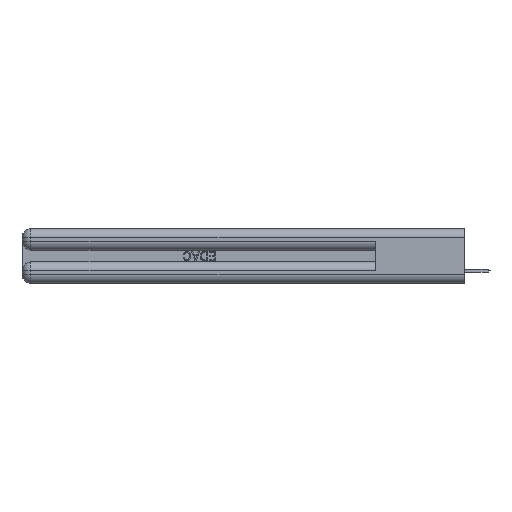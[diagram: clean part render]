
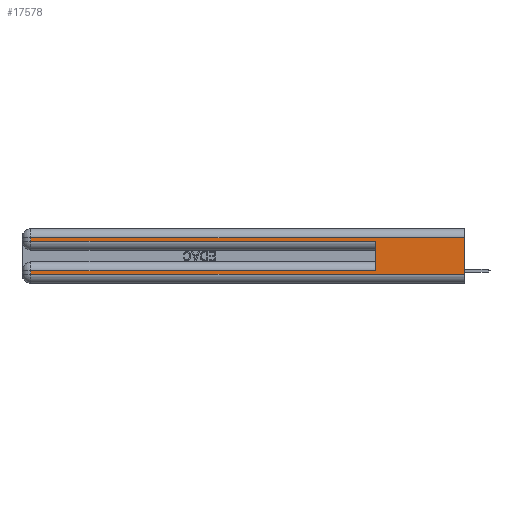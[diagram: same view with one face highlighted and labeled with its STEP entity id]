
A CAD part, left-side view. The second image highlights one B-rep face of the part: STEP entity #17578.
In plain terms, the highlighted planar face has unit normal (-1, 0, 0).
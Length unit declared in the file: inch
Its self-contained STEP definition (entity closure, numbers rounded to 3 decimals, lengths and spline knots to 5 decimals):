
#27 = VERTEX_POINT ( 'NONE', #25261 ) ;
#1653 = EDGE_CURVE ( 'NONE', #27, #19841, #10966, .T. ) ;
#1746 = EDGE_CURVE ( 'NONE', #1785, #27, #41986, .T. ) ;
#1785 = VERTEX_POINT ( 'NONE', #32756 ) ;
#2063 = VECTOR ( 'NONE', #39523, 39.37008 ) ;
#3125 = CARTESIAN_POINT ( 'NONE',  ( 0., 0., 0.06 ) ) ;
#3325 = DIRECTION ( 'NONE',  ( 0., 1., 0. ) ) ;
#3582 = CARTESIAN_POINT ( 'NONE',  ( 0., 0., 0.06 ) ) ;
#3936 = CARTESIAN_POINT ( 'NONE',  ( 0., 0., 0.31 ) ) ;
#4228 = EDGE_CURVE ( 'NONE', #26138, #29445, #43855, .T. ) ;
#4546 = FACE_OUTER_BOUND ( 'NONE', #14068, .T. ) ;
#5869 = CARTESIAN_POINT ( 'NONE',  ( 0., 0., 0.37 ) ) ;
#6634 = DIRECTION ( 'NONE',  ( 0., -1., 0. ) ) ;
#8595 = LINE ( 'NONE', #5869, #16922 ) ;
#8625 = CARTESIAN_POINT ( 'NONE',  ( 0., 0.6, 0.085 ) ) ;
#8633 = CARTESIAN_POINT ( 'NONE',  ( 0., 0., 0.285 ) ) ;
#8970 = VECTOR ( 'NONE', #6634, 39.37008 ) ;
#10349 = CARTESIAN_POINT ( 'NONE',  ( 0., 0.6, 0.145 ) ) ;
#10935 = ORIENTED_EDGE ( 'NONE', *, *, #47325, .T. ) ;
#10966 = LINE ( 'NONE', #22356, #48543 ) ;
#11278 = DIRECTION ( 'NONE',  ( 0., 0., -1. ) ) ;
#11519 = VECTOR ( 'NONE', #3325, 39.37008 ) ;
#12104 = LINE ( 'NONE', #36018, #2063 ) ;
#12710 = LINE ( 'NONE', #32894, #11519 ) ;
#13672 = VERTEX_POINT ( 'NONE', #29238 ) ;
#13933 = ORIENTED_EDGE ( 'NONE', *, *, #4228, .F. ) ;
#14068 = EDGE_LOOP ( 'NONE', ( #26017, #23106, #38516, #34493, #13933, #10935, #15301, #30255 ) ) ;
#14359 = LINE ( 'NONE', #3582, #8970 ) ;
#15072 = AXIS2_PLACEMENT_3D ( 'NONE', #21976, #41935, #11278 ) ;
#15301 = ORIENTED_EDGE ( 'NONE', *, *, #18560, .T. ) ;
#16390 = VECTOR ( 'NONE', #22319, 39.37008 ) ;
#16622 = EDGE_CURVE ( 'NONE', #19841, #29445, #30000, .T. ) ;
#16922 = VECTOR ( 'NONE', #24989, 39.37008 ) ;
#17297 = DIRECTION ( 'NONE',  ( 0., -1., 0. ) ) ;
#17509 = CARTESIAN_POINT ( 'NONE',  ( 0., 0.6, 0.285 ) ) ;
#17578 = ADVANCED_FACE ( 'NONE', ( #4546 ), #44819, .F. ) ;
#18560 = EDGE_CURVE ( 'NONE', #13672, #44566, #12104, .T. ) ;
#19841 = VERTEX_POINT ( 'NONE', #37607 ) ;
#19845 = VECTOR ( 'NONE', #17297, 39.37008 ) ;
#21607 = CARTESIAN_POINT ( 'NONE',  ( 0., 2.94, 0.06 ) ) ;
#21976 = CARTESIAN_POINT ( 'NONE',  ( 0., 0., 0.37 ) ) ;
#22319 = DIRECTION ( 'NONE',  ( 0., 0., 1. ) ) ;
#22356 = CARTESIAN_POINT ( 'NONE',  ( 0., 2.94, 0.37 ) ) ;
#23106 = ORIENTED_EDGE ( 'NONE', *, *, #1746, .T. ) ;
#23675 = VERTEX_POINT ( 'NONE', #3125 ) ;
#24989 = DIRECTION ( 'NONE',  ( 0., 0., -1. ) ) ;
#25261 = CARTESIAN_POINT ( 'NONE',  ( 0., 2.94, 0.31 ) ) ;
#26017 = ORIENTED_EDGE ( 'NONE', *, *, #29095, .F. ) ;
#26138 = VERTEX_POINT ( 'NONE', #8625 ) ;
#29095 = EDGE_CURVE ( 'NONE', #1785, #23675, #8595, .T. ) ;
#29238 = CARTESIAN_POINT ( 'NONE',  ( 0., 2.94, 0.085 ) ) ;
#29445 = VERTEX_POINT ( 'NONE', #17509 ) ;
#30000 = LINE ( 'NONE', #8633, #19845 ) ;
#30255 = ORIENTED_EDGE ( 'NONE', *, *, #42881, .T. ) ;
#32756 = CARTESIAN_POINT ( 'NONE',  ( 0., 0., 0.31 ) ) ;
#32894 = CARTESIAN_POINT ( 'NONE',  ( 0., 0., 0.085 ) ) ;
#33403 = DIRECTION ( 'NONE',  ( 0., 0., -1. ) ) ;
#34493 = ORIENTED_EDGE ( 'NONE', *, *, #16622, .T. ) ;
#34801 = VECTOR ( 'NONE', #39462, 39.37008 ) ;
#36018 = CARTESIAN_POINT ( 'NONE',  ( 0., 2.94, 0.37 ) ) ;
#37607 = CARTESIAN_POINT ( 'NONE',  ( 0., 2.94, 0.285 ) ) ;
#38516 = ORIENTED_EDGE ( 'NONE', *, *, #1653, .T. ) ;
#39462 = DIRECTION ( 'NONE',  ( 0., 1., 0. ) ) ;
#39523 = DIRECTION ( 'NONE',  ( 0., 0., -1. ) ) ;
#41935 = DIRECTION ( 'NONE',  ( 1., 0., 0. ) ) ;
#41986 = LINE ( 'NONE', #3936, #34801 ) ;
#42881 = EDGE_CURVE ( 'NONE', #44566, #23675, #14359, .T. ) ;
#43855 = LINE ( 'NONE', #10349, #16390 ) ;
#44566 = VERTEX_POINT ( 'NONE', #21607 ) ;
#44819 = PLANE ( 'NONE',  #15072 ) ;
#47325 = EDGE_CURVE ( 'NONE', #26138, #13672, #12710, .T. ) ;
#48543 = VECTOR ( 'NONE', #33403, 39.37008 ) ;
